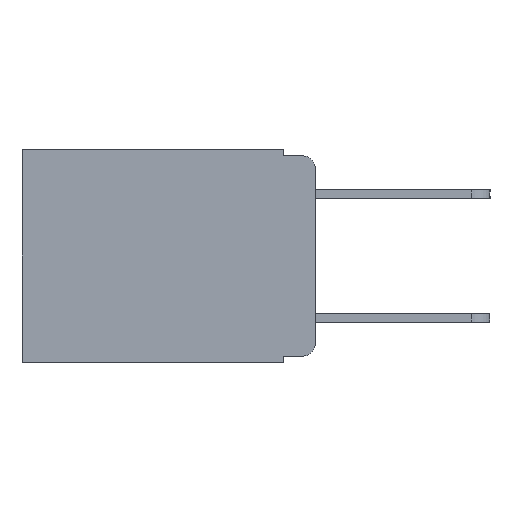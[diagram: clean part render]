
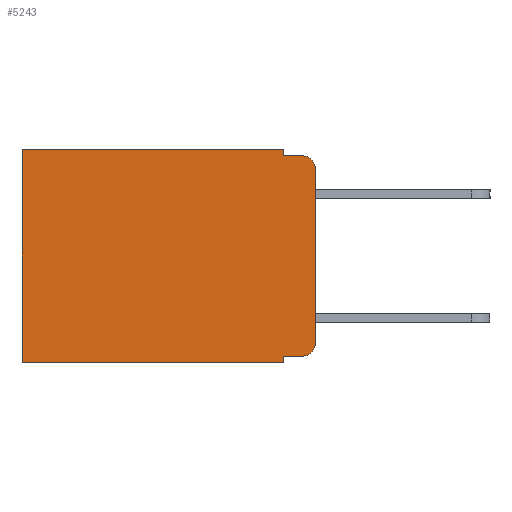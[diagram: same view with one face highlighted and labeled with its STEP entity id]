
A CAD part, left-side view. The second image highlights one B-rep face of the part: STEP entity #5243.
In plain terms, the highlighted planar face has unit normal (-1, 0, 0).
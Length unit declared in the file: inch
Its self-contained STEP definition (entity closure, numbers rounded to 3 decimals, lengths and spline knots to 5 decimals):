
#65 = VECTOR ( 'NONE', #1601, 39.37008 ) ;
#210 = DIRECTION ( 'NONE',  ( 0., 0., -1. ) ) ;
#232 = LINE ( 'NONE', #10505, #2267 ) ;
#367 = CARTESIAN_POINT ( 'NONE',  ( 0.298, 0.02, -0.333 ) ) ;
#530 = CARTESIAN_POINT ( 'NONE',  ( 0.298, 0.02, -0.03 ) ) ;
#605 = DIRECTION ( 'NONE',  ( 0., 1., 0. ) ) ;
#692 = AXIS2_PLACEMENT_3D ( 'NONE', #530, #5522, #210 ) ;
#820 = EDGE_CURVE ( 'NONE', #10193, #5031, #3060, .T. ) ;
#959 = CARTESIAN_POINT ( 'NONE',  ( 0.298, 0.473, -0.343 ) ) ;
#976 = FACE_OUTER_BOUND ( 'NONE', #9160, .T. ) ;
#1549 = EDGE_CURVE ( 'NONE', #5077, #4304, #5678, .T. ) ;
#1601 = DIRECTION ( 'NONE',  ( 0., 0., -1. ) ) ;
#1836 = EDGE_CURVE ( 'NONE', #8741, #5031, #3599, .T. ) ;
#2267 = VECTOR ( 'NONE', #6579, 39.37008 ) ;
#2268 = CARTESIAN_POINT ( 'NONE',  ( 0.298, 0.051, 0. ) ) ;
#2398 = ORIENTED_EDGE ( 'NONE', *, *, #8537, .F. ) ;
#2408 = VECTOR ( 'NONE', #2671, 39.37008 ) ;
#2466 = ORIENTED_EDGE ( 'NONE', *, *, #8913, .F. ) ;
#2671 = DIRECTION ( 'NONE',  ( 0., 1., 0. ) ) ;
#2686 = EDGE_CURVE ( 'NONE', #8488, #7618, #9084, .T. ) ;
#2793 = ORIENTED_EDGE ( 'NONE', *, *, #6383, .T. ) ;
#3053 = DIRECTION ( 'NONE',  ( 0., -1., 0. ) ) ;
#3060 = LINE ( 'NONE', #9146, #5113 ) ;
#3165 = EDGE_CURVE ( 'NONE', #10105, #3390, #9311, .T. ) ;
#3265 = CARTESIAN_POINT ( 'NONE',  ( 0.298, 0., -0.343 ) ) ;
#3316 = VECTOR ( 'NONE', #605, 39.37008 ) ;
#3390 = VERTEX_POINT ( 'NONE', #367 ) ;
#3392 = VERTEX_POINT ( 'NONE', #10584 ) ;
#3546 = CARTESIAN_POINT ( 'NONE',  ( 0.298, 0.473, 0. ) ) ;
#3599 = CIRCLE ( 'NONE', #692, 0.02 ) ;
#3774 = ORIENTED_EDGE ( 'NONE', *, *, #8006, .F. ) ;
#3891 = CARTESIAN_POINT ( 'NONE',  ( 0.298, 0.051, -0.343 ) ) ;
#4304 = VERTEX_POINT ( 'NONE', #3546 ) ;
#4618 = AXIS2_PLACEMENT_3D ( 'NONE', #9390, #9439, #5020 ) ;
#4913 = CARTESIAN_POINT ( 'NONE',  ( 0.298, 0., 0. ) ) ;
#5020 = DIRECTION ( 'NONE',  ( 0., 0., -1. ) ) ;
#5031 = VERTEX_POINT ( 'NONE', #8034 ) ;
#5062 = AXIS2_PLACEMENT_3D ( 'NONE', #10043, #10053, #9943 ) ;
#5077 = VERTEX_POINT ( 'NONE', #2268 ) ;
#5113 = VECTOR ( 'NONE', #3053, 39.37008 ) ;
#5243 = ADVANCED_FACE ( 'NONE', ( #976 ), #9172, .F. ) ;
#5522 = DIRECTION ( 'NONE',  ( -1., 0., 0. ) ) ;
#5678 = LINE ( 'NONE', #7791, #3316 ) ;
#5900 = DIRECTION ( 'NONE',  ( 0., 0., -1. ) ) ;
#6383 = EDGE_CURVE ( 'NONE', #3390, #3392, #10201, .T. ) ;
#6579 = DIRECTION ( 'NONE',  ( 0., 0., -1. ) ) ;
#6932 = CARTESIAN_POINT ( 'NONE',  ( 0.298, 0.051, -0.333 ) ) ;
#6998 = VECTOR ( 'NONE', #5900, 39.37008 ) ;
#7106 = EDGE_CURVE ( 'NONE', #4304, #7618, #9333, .T. ) ;
#7231 = VECTOR ( 'NONE', #8849, 39.37008 ) ;
#7450 = CARTESIAN_POINT ( 'NONE',  ( 0.298, 0., -0.03 ) ) ;
#7618 = VERTEX_POINT ( 'NONE', #959 ) ;
#7759 = DIRECTION ( 'NONE',  ( 0., 0., -1. ) ) ;
#7791 = CARTESIAN_POINT ( 'NONE',  ( 0.298, 0., 0. ) ) ;
#8006 = EDGE_CURVE ( 'NONE', #5077, #10193, #232, .T. ) ;
#8034 = CARTESIAN_POINT ( 'NONE',  ( 0.298, 0.02, -0.01 ) ) ;
#8259 = CARTESIAN_POINT ( 'NONE',  ( 0.298, 0.473, 0. ) ) ;
#8488 = VERTEX_POINT ( 'NONE', #3891 ) ;
#8537 = EDGE_CURVE ( 'NONE', #8741, #3392, #9062, .T. ) ;
#8561 = ORIENTED_EDGE ( 'NONE', *, *, #1836, .T. ) ;
#8615 = CARTESIAN_POINT ( 'NONE',  ( 0.298, 0.051, -0.333 ) ) ;
#8741 = VERTEX_POINT ( 'NONE', #7450 ) ;
#8819 = VECTOR ( 'NONE', #7759, 39.37008 ) ;
#8849 = DIRECTION ( 'NONE',  ( 0., -1., 0. ) ) ;
#8913 = EDGE_CURVE ( 'NONE', #10105, #8488, #9288, .T. ) ;
#8938 = CARTESIAN_POINT ( 'NONE',  ( 0.298, 0.051, -0.01 ) ) ;
#9019 = ORIENTED_EDGE ( 'NONE', *, *, #7106, .T. ) ;
#9062 = LINE ( 'NONE', #4913, #8819 ) ;
#9084 = LINE ( 'NONE', #3265, #2408 ) ;
#9146 = CARTESIAN_POINT ( 'NONE',  ( 0.298, 0.051, -0.01 ) ) ;
#9160 = EDGE_LOOP ( 'NONE', ( #2398, #8561, #10284, #3774, #10618, #9019, #10065, #2466, #9902, #2793 ) ) ;
#9172 = PLANE ( 'NONE',  #4618 ) ;
#9278 = CARTESIAN_POINT ( 'NONE',  ( 0.298, 0.051, 0. ) ) ;
#9288 = LINE ( 'NONE', #9278, #65 ) ;
#9311 = LINE ( 'NONE', #6932, #7231 ) ;
#9333 = LINE ( 'NONE', #8259, #6998 ) ;
#9390 = CARTESIAN_POINT ( 'NONE',  ( 0.298, 0., 0. ) ) ;
#9439 = DIRECTION ( 'NONE',  ( 1., 0., 0. ) ) ;
#9902 = ORIENTED_EDGE ( 'NONE', *, *, #3165, .T. ) ;
#9943 = DIRECTION ( 'NONE',  ( 0., 0., -1. ) ) ;
#10043 = CARTESIAN_POINT ( 'NONE',  ( 0.298, 0.02, -0.313 ) ) ;
#10053 = DIRECTION ( 'NONE',  ( -1., 0., 0. ) ) ;
#10065 = ORIENTED_EDGE ( 'NONE', *, *, #2686, .F. ) ;
#10105 = VERTEX_POINT ( 'NONE', #8615 ) ;
#10193 = VERTEX_POINT ( 'NONE', #8938 ) ;
#10201 = CIRCLE ( 'NONE', #5062, 0.02 ) ;
#10284 = ORIENTED_EDGE ( 'NONE', *, *, #820, .F. ) ;
#10505 = CARTESIAN_POINT ( 'NONE',  ( 0.298, 0.051, 0. ) ) ;
#10584 = CARTESIAN_POINT ( 'NONE',  ( 0.298, 0., -0.313 ) ) ;
#10618 = ORIENTED_EDGE ( 'NONE', *, *, #1549, .T. ) ;
